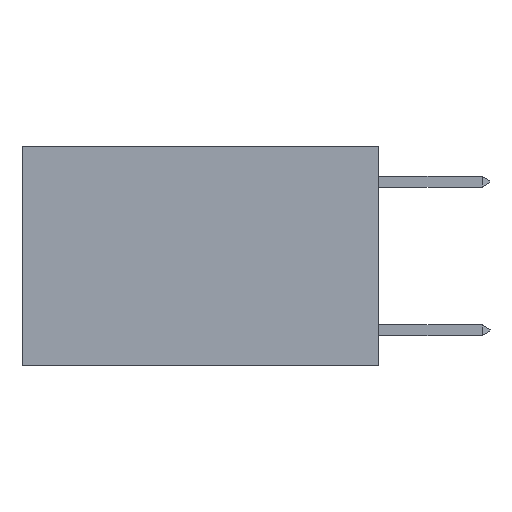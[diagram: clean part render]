
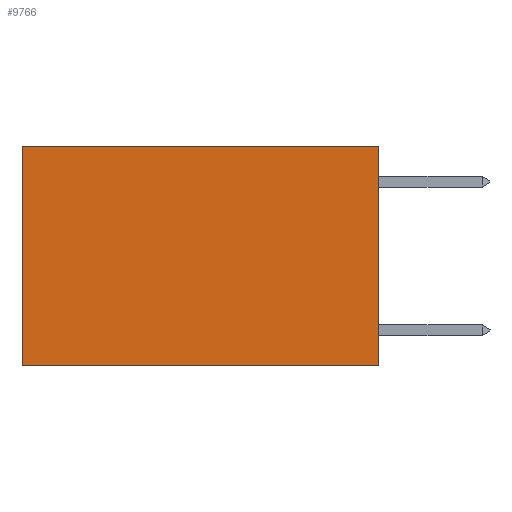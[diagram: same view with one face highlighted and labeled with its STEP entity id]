
A CAD part, left-side view. The second image highlights one B-rep face of the part: STEP entity #9766.
In plain terms, the highlighted planar face has unit normal (-1, 0, 0).
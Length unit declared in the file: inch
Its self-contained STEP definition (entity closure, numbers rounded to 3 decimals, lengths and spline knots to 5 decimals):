
#34 = DIRECTION ( 'NONE',  ( 1., 0., 0. ) ) ;
#555 = VECTOR ( 'NONE', #2253, 39.37008 ) ;
#807 = VERTEX_POINT ( 'NONE', #1478 ) ;
#881 = ORIENTED_EDGE ( 'NONE', *, *, #3627, .F. ) ;
#1289 = VECTOR ( 'NONE', #8251, 39.37008 ) ;
#1478 = CARTESIAN_POINT ( 'NONE',  ( 0.2625, 0., -0.37 ) ) ;
#1519 = LINE ( 'NONE', #5770, #8075 ) ;
#1851 = VECTOR ( 'NONE', #9210, 39.37008 ) ;
#2253 = DIRECTION ( 'NONE',  ( 0., 1., 0. ) ) ;
#2863 = EDGE_CURVE ( 'NONE', #4464, #807, #10626, .T. ) ;
#3627 = EDGE_CURVE ( 'NONE', #807, #5664, #4191, .T. ) ;
#3756 = ORIENTED_EDGE ( 'NONE', *, *, #2863, .F. ) ;
#4191 = LINE ( 'NONE', #9415, #1851 ) ;
#4302 = CARTESIAN_POINT ( 'NONE',  ( 0.2625, 0.6, -0.37 ) ) ;
#4464 = VERTEX_POINT ( 'NONE', #10650 ) ;
#4657 = PLANE ( 'NONE',  #7721 ) ;
#5664 = VERTEX_POINT ( 'NONE', #4302 ) ;
#5770 = CARTESIAN_POINT ( 'NONE',  ( 0.2625, 0.6, 0. ) ) ;
#5806 = CARTESIAN_POINT ( 'NONE',  ( 0.2625, 0., 0. ) ) ;
#6177 = EDGE_CURVE ( 'NONE', #6540, #5664, #1519, .T. ) ;
#6206 = FACE_OUTER_BOUND ( 'NONE', #11079, .T. ) ;
#6236 = EDGE_CURVE ( 'NONE', #4464, #6540, #10085, .T. ) ;
#6451 = DIRECTION ( 'NONE',  ( 0., 0., -1. ) ) ;
#6540 = VERTEX_POINT ( 'NONE', #7872 ) ;
#7438 = ORIENTED_EDGE ( 'NONE', *, *, #6236, .T. ) ;
#7496 = ORIENTED_EDGE ( 'NONE', *, *, #6177, .T. ) ;
#7721 = AXIS2_PLACEMENT_3D ( 'NONE', #10703, #34, #6451 ) ;
#7872 = CARTESIAN_POINT ( 'NONE',  ( 0.2625, 0.6, 0. ) ) ;
#8075 = VECTOR ( 'NONE', #8410, 39.37008 ) ;
#8251 = DIRECTION ( 'NONE',  ( 0., 0., -1. ) ) ;
#8410 = DIRECTION ( 'NONE',  ( 0., 0., -1. ) ) ;
#9210 = DIRECTION ( 'NONE',  ( 0., 1., 0. ) ) ;
#9415 = CARTESIAN_POINT ( 'NONE',  ( 0.2625, 0., -0.37 ) ) ;
#9766 = ADVANCED_FACE ( 'NONE', ( #6206 ), #4657, .F. ) ;
#10085 = LINE ( 'NONE', #5806, #555 ) ;
#10144 = CARTESIAN_POINT ( 'NONE',  ( 0.2625, 0., 0. ) ) ;
#10626 = LINE ( 'NONE', #10144, #1289 ) ;
#10650 = CARTESIAN_POINT ( 'NONE',  ( 0.2625, 0., 0. ) ) ;
#10703 = CARTESIAN_POINT ( 'NONE',  ( 0.2625, 0., 0. ) ) ;
#11079 = EDGE_LOOP ( 'NONE', ( #7496, #881, #3756, #7438 ) ) ;
